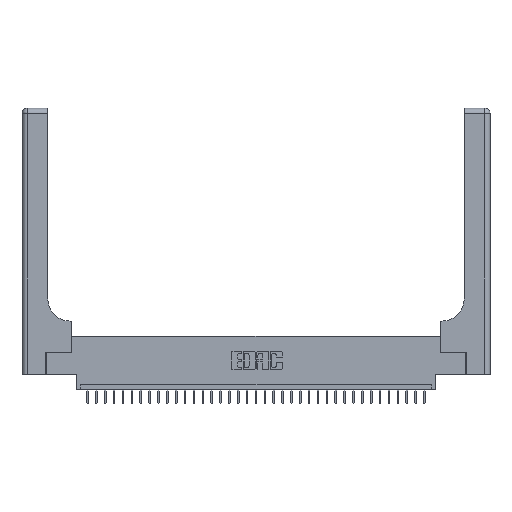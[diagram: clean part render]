
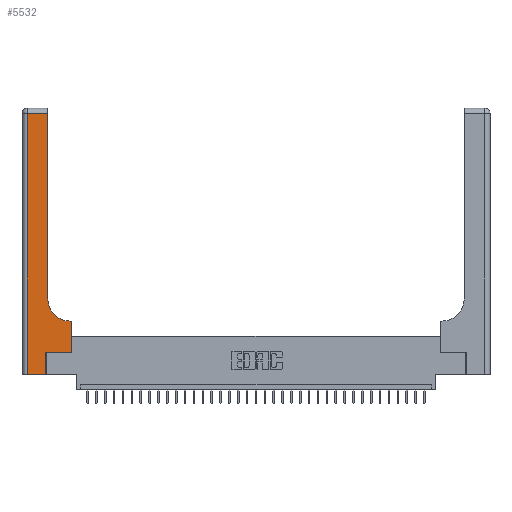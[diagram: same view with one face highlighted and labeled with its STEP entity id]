
A CAD part, top view. The second image highlights one B-rep face of the part: STEP entity #5532.
In plain terms, the highlighted planar face has unit normal (0, 0, 1).
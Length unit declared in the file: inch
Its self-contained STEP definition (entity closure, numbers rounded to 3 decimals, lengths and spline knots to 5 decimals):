
#110 = EDGE_CURVE ( 'NONE', #25017, #3862, #7014, .T. ) ;
#830 = LINE ( 'NONE', #2763, #10255 ) ;
#1137 = EDGE_CURVE ( 'NONE', #5028, #22704, #3576, .T. ) ;
#2208 = LINE ( 'NONE', #19698, #23059 ) ;
#2756 = VECTOR ( 'NONE', #3270, 39.37008 ) ;
#2763 = CARTESIAN_POINT ( 'NONE',  ( 0.06, 3., 0.37 ) ) ;
#3270 = DIRECTION ( 'NONE',  ( 0., 1., 0. ) ) ;
#3458 = VERTEX_POINT ( 'NONE', #8171 ) ;
#3576 = LINE ( 'NONE', #25271, #2756 ) ;
#3862 = VERTEX_POINT ( 'NONE', #8359 ) ;
#3961 = EDGE_CURVE ( 'NONE', #17828, #4338, #16237, .T. ) ;
#4305 = ORIENTED_EDGE ( 'NONE', *, *, #3961, .T. ) ;
#4338 = VERTEX_POINT ( 'NONE', #19952 ) ;
#4579 = VECTOR ( 'NONE', #10491, 39.37008 ) ;
#4727 = ORIENTED_EDGE ( 'NONE', *, *, #110, .T. ) ;
#5028 = VERTEX_POINT ( 'NONE', #18557 ) ;
#5532 = ADVANCED_FACE ( 'NONE', ( #16114 ), #32880, .F. ) ;
#6412 = EDGE_CURVE ( 'NONE', #3862, #19154, #34248, .T. ) ;
#7014 = LINE ( 'NONE', #19236, #7893 ) ;
#7037 = VECTOR ( 'NONE', #31728, 39.37008 ) ;
#7316 = VECTOR ( 'NONE', #30881, 39.37008 ) ;
#7893 = VECTOR ( 'NONE', #23170, 39.37008 ) ;
#8171 = CARTESIAN_POINT ( 'NONE',  ( 0.5415, 0.6, 0.37 ) ) ;
#8359 = CARTESIAN_POINT ( 'NONE',  ( 0.2915, 2.94, 0.37 ) ) ;
#9250 = EDGE_CURVE ( 'NONE', #3458, #25017, #24365, .T. ) ;
#9414 = ORIENTED_EDGE ( 'NONE', *, *, #11395, .T. ) ;
#10255 = VECTOR ( 'NONE', #29450, 39.37008 ) ;
#10491 = DIRECTION ( 'NONE',  ( -1., 0., 0. ) ) ;
#11065 = DIRECTION ( 'NONE',  ( -1., 0., 0. ) ) ;
#11395 = EDGE_CURVE ( 'NONE', #4338, #3458, #19923, .T. ) ;
#12293 = CARTESIAN_POINT ( 'NONE',  ( 0.2915, 0.6, 0.37 ) ) ;
#12536 = CARTESIAN_POINT ( 'NONE',  ( 0.2915, 0.85, 0.37 ) ) ;
#13190 = ORIENTED_EDGE ( 'NONE', *, *, #15072, .T. ) ;
#13410 = AXIS2_PLACEMENT_3D ( 'NONE', #14298, #19393, #11065 ) ;
#13558 = DIRECTION ( 'NONE',  ( 0., 1., 0. ) ) ;
#13888 = ORIENTED_EDGE ( 'NONE', *, *, #22702, .T. ) ;
#14298 = CARTESIAN_POINT ( 'NONE',  ( 0., 3., 0.37 ) ) ;
#15072 = EDGE_CURVE ( 'NONE', #22704, #17828, #33661, .T. ) ;
#16114 = FACE_OUTER_BOUND ( 'NONE', #29277, .T. ) ;
#16220 = CARTESIAN_POINT ( 'NONE',  ( 0., 2.94, 0.37 ) ) ;
#16237 = LINE ( 'NONE', #29792, #31880 ) ;
#17456 = CARTESIAN_POINT ( 'NONE',  ( 0.5415, 0.85, 0.37 ) ) ;
#17828 = VERTEX_POINT ( 'NONE', #27914 ) ;
#18557 = CARTESIAN_POINT ( 'NONE',  ( 0.269, 0., 0.37 ) ) ;
#19154 = VERTEX_POINT ( 'NONE', #21611 ) ;
#19236 = CARTESIAN_POINT ( 'NONE',  ( 0.2915, 3., 0.37 ) ) ;
#19393 = DIRECTION ( 'NONE',  ( 0., 0., -1. ) ) ;
#19454 = DIRECTION ( 'NONE',  ( 1., 0., 0. ) ) ;
#19698 = CARTESIAN_POINT ( 'NONE',  ( 0., 0., 0.37 ) ) ;
#19892 = CARTESIAN_POINT ( 'NONE',  ( 0.269, 0.25, 0.37 ) ) ;
#19923 = LINE ( 'NONE', #12293, #4579 ) ;
#19952 = CARTESIAN_POINT ( 'NONE',  ( 0.5585, 0.6, 0.37 ) ) ;
#21611 = CARTESIAN_POINT ( 'NONE',  ( 0.06, 2.94, 0.37 ) ) ;
#22191 = CARTESIAN_POINT ( 'NONE',  ( 0.269, 0.25, 0.37 ) ) ;
#22702 = EDGE_CURVE ( 'NONE', #23033, #5028, #2208, .T. ) ;
#22704 = VERTEX_POINT ( 'NONE', #22191 ) ;
#23033 = VERTEX_POINT ( 'NONE', #28304 ) ;
#23059 = VECTOR ( 'NONE', #19454, 39.37008 ) ;
#23170 = DIRECTION ( 'NONE',  ( 0., 1., 0. ) ) ;
#24000 = ORIENTED_EDGE ( 'NONE', *, *, #6412, .T. ) ;
#24365 = CIRCLE ( 'NONE', #32737, 0.25 ) ;
#25017 = VERTEX_POINT ( 'NONE', #12536 ) ;
#25105 = ORIENTED_EDGE ( 'NONE', *, *, #1137, .T. ) ;
#25271 = CARTESIAN_POINT ( 'NONE',  ( 0.269, 0., 0.37 ) ) ;
#26112 = ORIENTED_EDGE ( 'NONE', *, *, #9250, .T. ) ;
#27914 = CARTESIAN_POINT ( 'NONE',  ( 0.5585, 0.25, 0.37 ) ) ;
#28304 = CARTESIAN_POINT ( 'NONE',  ( 0.06, 0., 0.37 ) ) ;
#28426 = DIRECTION ( 'NONE',  ( 1., 0., 0. ) ) ;
#29277 = EDGE_LOOP ( 'NONE', ( #4727, #24000, #30076, #13888, #25105, #13190, #4305, #9414, #26112 ) ) ;
#29450 = DIRECTION ( 'NONE',  ( 0., -1., 0. ) ) ;
#29792 = CARTESIAN_POINT ( 'NONE',  ( 0.5585, 0.25, 0.37 ) ) ;
#30076 = ORIENTED_EDGE ( 'NONE', *, *, #34525, .T. ) ;
#30881 = DIRECTION ( 'NONE',  ( 1., 0., 0. ) ) ;
#31037 = DIRECTION ( 'NONE',  ( 0., 0., -1. ) ) ;
#31728 = DIRECTION ( 'NONE',  ( -1., 0., 0. ) ) ;
#31880 = VECTOR ( 'NONE', #13558, 39.37008 ) ;
#32737 = AXIS2_PLACEMENT_3D ( 'NONE', #17456, #31037, #28426 ) ;
#32880 = PLANE ( 'NONE',  #13410 ) ;
#33661 = LINE ( 'NONE', #19892, #7316 ) ;
#34248 = LINE ( 'NONE', #16220, #7037 ) ;
#34525 = EDGE_CURVE ( 'NONE', #19154, #23033, #830, .T. ) ;
